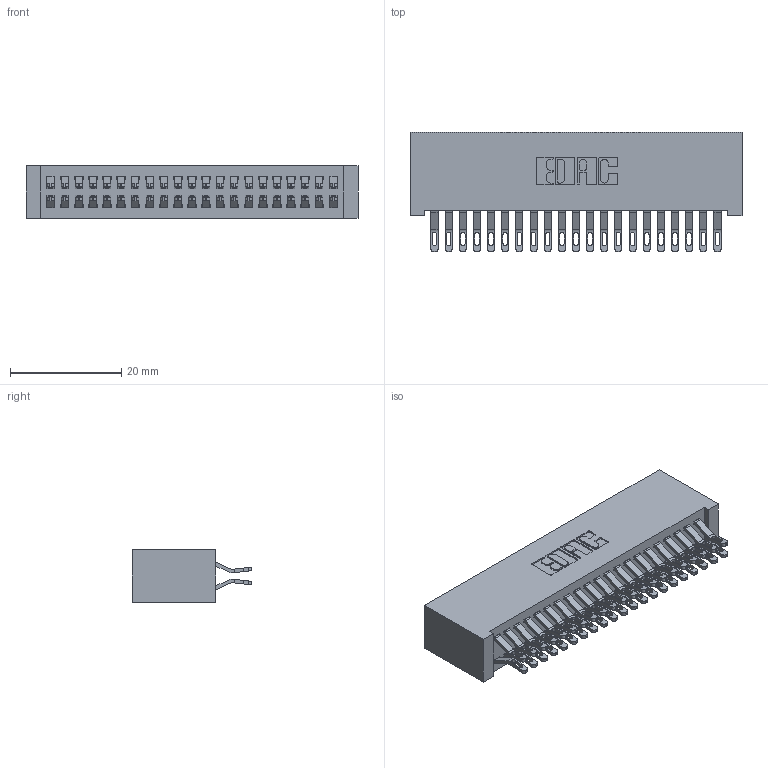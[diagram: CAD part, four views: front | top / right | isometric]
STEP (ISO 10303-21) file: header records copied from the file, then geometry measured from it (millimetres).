
FILE_DESCRIPTION (( 'STEP AP203' ), '1' );
FILE_NAME ('392-042-555-201.STEP', '2019-10-07T21:19:34', ( '' ), ( '' ), 'SwSTEP 2.0', 'SolidWorks 2016', '' );
FILE_SCHEMA (( 'CONFIG_CONTROL_DESIGN' ));
Length unit declared in the file: inch
Products named in the file (3): 342 Part_Lugless; 345-292-001_555 Tail; 392-042-555-201
Assembly tree (43 placements, depth 2):
  392-042-555-201
    342 Part_Lugless
    345-292-001_555 Tail  x42
Bounding box: 59.59 x 21.47 x 9.4 mm (x, y, z)
Volume: 5810.8 mm3; surface area: 9793.7 mm2
Topology: 43 solids, 43 shells, 2538 faces, 7961 edges, 5306 vertices
Faces by surface type: plane 1490, cylinder 1048
Entity records: 16143 total; most frequent: CARTESIAN_POINT 2732, ORIENTED_EDGE 2638, DIRECTION 2335, EDGE_CURVE 1319, LINE 1179, VECTOR 1179, VERTEX_POINT 878, AXIS2_PLACEMENT_3D 578
